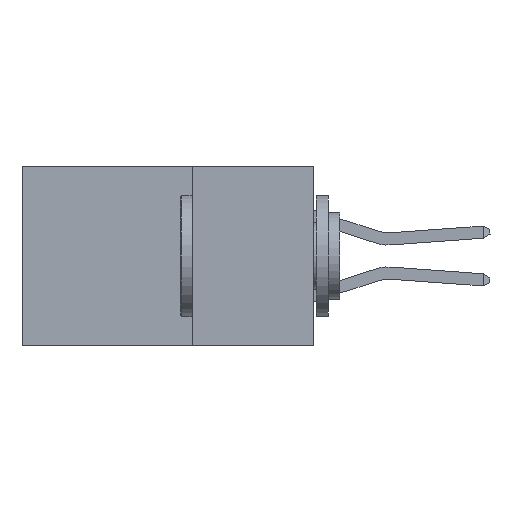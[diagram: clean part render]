
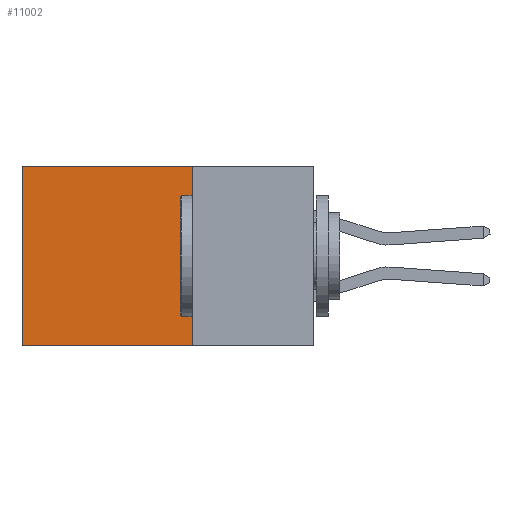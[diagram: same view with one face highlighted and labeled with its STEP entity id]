
A CAD part, left-side view. The second image highlights one B-rep face of the part: STEP entity #11002.
In plain terms, the highlighted planar face has unit normal (-1, 0, 0).
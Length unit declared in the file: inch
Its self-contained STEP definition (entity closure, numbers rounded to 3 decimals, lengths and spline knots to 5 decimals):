
#106 = VECTOR ( 'NONE', #8245, 39.37008 ) ;
#289 = VERTEX_POINT ( 'NONE', #40841 ) ;
#1962 = ORIENTED_EDGE ( 'NONE', *, *, #11877, .T. ) ;
#5021 = ORIENTED_EDGE ( 'NONE', *, *, #12981, .T. ) ;
#5237 = CARTESIAN_POINT ( 'NONE',  ( 0.2875, 0.6, -0.37 ) ) ;
#5377 = ORIENTED_EDGE ( 'NONE', *, *, #25938, .F. ) ;
#5531 = VECTOR ( 'NONE', #37259, 39.37008 ) ;
#7321 = VERTEX_POINT ( 'NONE', #5237 ) ;
#8245 = DIRECTION ( 'NONE',  ( 0., 1., 0. ) ) ;
#8571 = VERTEX_POINT ( 'NONE', #37693 ) ;
#11002 = ADVANCED_FACE ( 'NONE', ( #12608 ), #20988, .F. ) ;
#11145 = CARTESIAN_POINT ( 'NONE',  ( 0.2875, 0.25, 0. ) ) ;
#11877 = EDGE_CURVE ( 'NONE', #289, #8571, #36621, .T. ) ;
#12608 = FACE_OUTER_BOUND ( 'NONE', #40414, .T. ) ;
#12981 = EDGE_CURVE ( 'NONE', #8571, #7321, #13573, .T. ) ;
#13573 = LINE ( 'NONE', #34002, #5531 ) ;
#14216 = EDGE_CURVE ( 'NONE', #289, #38009, #24284, .T. ) ;
#15518 = VECTOR ( 'NONE', #35422, 39.37008 ) ;
#16814 = ORIENTED_EDGE ( 'NONE', *, *, #14216, .F. ) ;
#20988 = PLANE ( 'NONE',  #37796 ) ;
#21133 = DIRECTION ( 'NONE',  ( 0., 0., -1. ) ) ;
#22408 = CARTESIAN_POINT ( 'NONE',  ( 0.2875, 0.25, -0.37 ) ) ;
#24284 = LINE ( 'NONE', #32170, #15518 ) ;
#25938 = EDGE_CURVE ( 'NONE', #38009, #7321, #34451, .T. ) ;
#27992 = VECTOR ( 'NONE', #29131, 39.37008 ) ;
#28110 = CARTESIAN_POINT ( 'NONE',  ( 0.2875, 0.25, -0.37 ) ) ;
#29131 = DIRECTION ( 'NONE',  ( 0., 1., 0. ) ) ;
#32170 = CARTESIAN_POINT ( 'NONE',  ( 0.2875, 0.25, 0. ) ) ;
#34002 = CARTESIAN_POINT ( 'NONE',  ( 0.2875, 0.6, 0. ) ) ;
#34451 = LINE ( 'NONE', #28110, #106 ) ;
#35422 = DIRECTION ( 'NONE',  ( 0., 0., -1. ) ) ;
#36621 = LINE ( 'NONE', #41976, #27992 ) ;
#37259 = DIRECTION ( 'NONE',  ( 0., 0., -1. ) ) ;
#37693 = CARTESIAN_POINT ( 'NONE',  ( 0.2875, 0.6, 0. ) ) ;
#37796 = AXIS2_PLACEMENT_3D ( 'NONE', #11145, #40626, #21133 ) ;
#38009 = VERTEX_POINT ( 'NONE', #22408 ) ;
#40414 = EDGE_LOOP ( 'NONE', ( #5021, #5377, #16814, #1962 ) ) ;
#40626 = DIRECTION ( 'NONE',  ( 1., 0., 0. ) ) ;
#40841 = CARTESIAN_POINT ( 'NONE',  ( 0.2875, 0.25, 0. ) ) ;
#41976 = CARTESIAN_POINT ( 'NONE',  ( 0.2875, 0.25, 0. ) ) ;
